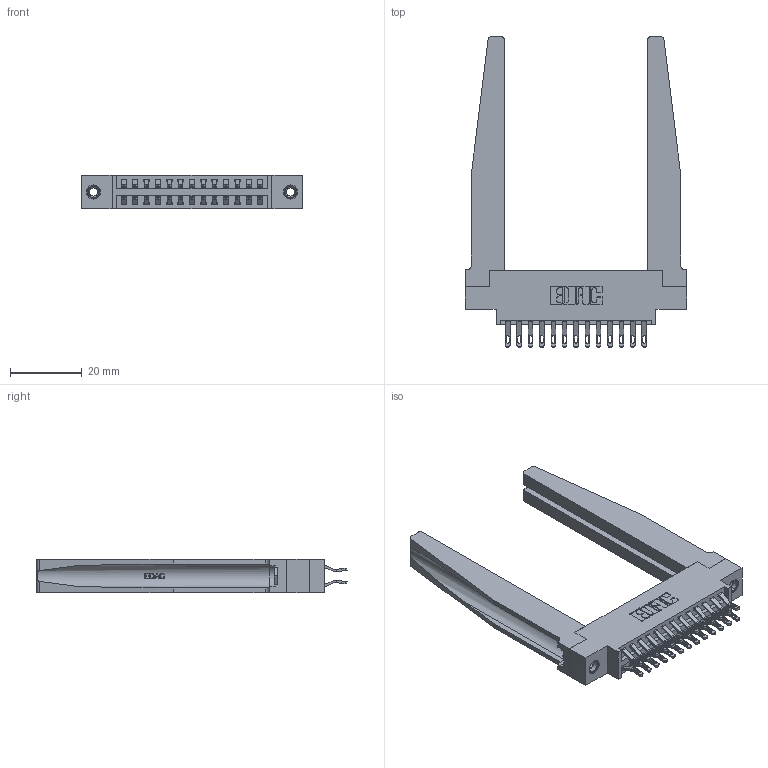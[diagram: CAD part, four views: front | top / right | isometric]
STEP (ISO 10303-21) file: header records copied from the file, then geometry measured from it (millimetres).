
FILE_DESCRIPTION (( 'STEP AP203' ), '1' );
FILE_NAME ('346-026-555-878.STEP', '2022-05-19T02:26:21', ( '' ), ( '' ), 'SwSTEP 2.0', 'SolidWorks 2020', '' );
FILE_SCHEMA (( 'CONFIG_CONTROL_DESIGN' ));
Length unit declared in the file: inch
Products named in the file (5): 346 Part_0.170 Offset - 0.156 Dia-TH; 346-026-555-878; 346-220-078_345-220-078; 345-292-001_555 Tail; 345-250-001_345-250-001-102
Assembly tree (31 placements, depth 2):
  346-026-555-878
    346 Part_0.170 Offset - 0.156 Dia-TH
    345-292-001_555 Tail  x26
    346-220-078_345-220-078  x2
    345-250-001_345-250-001-102  x2
Bounding box: 61.85 x 86.74 x 9.4 mm (x, y, z)
Volume: 12617.4 mm3; surface area: 14411.4 mm2
Topology: 31 solids, 31 shells, 1882 faces, 5743 edges, 3818 vertices
Faces by surface type: plane 1094, cylinder 736, bspline 36, cone 12, torus 4
Entity records: 18010 total; most frequent: CARTESIAN_POINT 3987, ORIENTED_EDGE 2778, DIRECTION 2519, EDGE_CURVE 1389, LINE 1091, VECTOR 1091, VERTEX_POINT 920, AXIS2_PLACEMENT_3D 714
